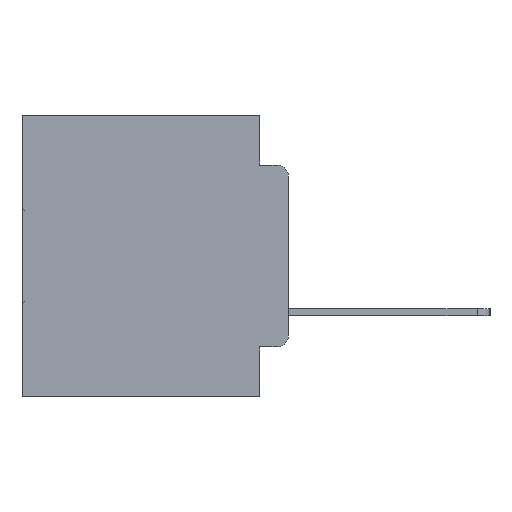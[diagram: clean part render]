
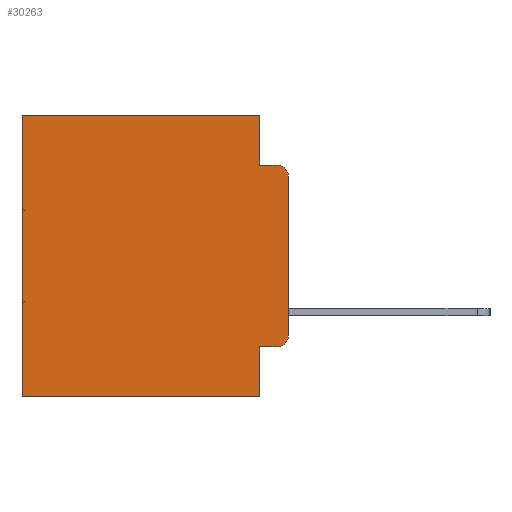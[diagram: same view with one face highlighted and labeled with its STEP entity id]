
A CAD part, left-side view. The second image highlights one B-rep face of the part: STEP entity #30263.
In plain terms, the highlighted planar face has unit normal (-1, 0, 0).
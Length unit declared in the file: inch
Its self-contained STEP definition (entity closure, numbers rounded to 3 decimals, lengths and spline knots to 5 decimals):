
#615 = ORIENTED_EDGE ( 'NONE', *, *, #15617, .T. ) ;
#958 = CARTESIAN_POINT ( 'NONE',  ( 0.298, 0.051, -0.5 ) ) ;
#1130 = VERTEX_POINT ( 'NONE', #10493 ) ;
#1431 = DIRECTION ( 'NONE',  ( 0., -1., 0. ) ) ;
#2017 = EDGE_CURVE ( 'NONE', #1130, #23498, #22075, .T. ) ;
#2206 = ORIENTED_EDGE ( 'NONE', *, *, #25310, .F. ) ;
#2892 = CARTESIAN_POINT ( 'NONE',  ( 0.298, 0.473, -0.5 ) ) ;
#2958 = LINE ( 'NONE', #23111, #21338 ) ;
#3974 = DIRECTION ( 'NONE',  ( 0., 1., 0. ) ) ;
#4320 = VERTEX_POINT ( 'NONE', #21616 ) ;
#4797 = VERTEX_POINT ( 'NONE', #20973 ) ;
#5400 = EDGE_CURVE ( 'NONE', #9654, #25665, #5758, .T. ) ;
#5598 = LINE ( 'NONE', #24920, #23890 ) ;
#5651 = ORIENTED_EDGE ( 'NONE', *, *, #16814, .T. ) ;
#5758 = LINE ( 'NONE', #22285, #17746 ) ;
#5810 = LINE ( 'NONE', #27133, #11495 ) ;
#5849 = DIRECTION ( 'NONE',  ( 0., 0., -1. ) ) ;
#6134 = LINE ( 'NONE', #29048, #24399 ) ;
#6299 = EDGE_CURVE ( 'NONE', #27684, #7325, #24722, .T. ) ;
#7325 = VERTEX_POINT ( 'NONE', #17608 ) ;
#7458 = EDGE_CURVE ( 'NONE', #14294, #4320, #10223, .T. ) ;
#7907 = ORIENTED_EDGE ( 'NONE', *, *, #7458, .F. ) ;
#7931 = EDGE_CURVE ( 'NONE', #11398, #27684, #5598, .T. ) ;
#8004 = DIRECTION ( 'NONE',  ( 0., 0., -1. ) ) ;
#8019 = CARTESIAN_POINT ( 'NONE',  ( 0.298, 0., -0.1085 ) ) ;
#8053 = EDGE_CURVE ( 'NONE', #4797, #4320, #20947, .T. ) ;
#8425 = DIRECTION ( 'NONE',  ( 0., 0., -1. ) ) ;
#9654 = VERTEX_POINT ( 'NONE', #12710 ) ;
#10223 = LINE ( 'NONE', #20423, #28418 ) ;
#10296 = EDGE_LOOP ( 'NONE', ( #7907, #615, #12493, #17296, #15074, #13600, #2206, #22820, #5651, #21004 ) ) ;
#10493 = CARTESIAN_POINT ( 'NONE',  ( 0.298, 0.051, -0.4115 ) ) ;
#10593 = DIRECTION ( 'NONE',  ( -1., 0., 0. ) ) ;
#10696 = AXIS2_PLACEMENT_3D ( 'NONE', #27772, #13616, #30148 ) ;
#11390 = VECTOR ( 'NONE', #1431, 39.37008 ) ;
#11398 = VERTEX_POINT ( 'NONE', #12639 ) ;
#11495 = VECTOR ( 'NONE', #22474, 39.37008 ) ;
#11769 = PLANE ( 'NONE',  #27944 ) ;
#11866 = DIRECTION ( 'NONE',  ( 0., 0., -1. ) ) ;
#12493 = ORIENTED_EDGE ( 'NONE', *, *, #6299, .F. ) ;
#12639 = CARTESIAN_POINT ( 'NONE',  ( 0.298, 0.051, 0. ) ) ;
#12710 = CARTESIAN_POINT ( 'NONE',  ( 0.298, 0.473, 0. ) ) ;
#13374 = CARTESIAN_POINT ( 'NONE',  ( 0.298, 0.051, -0.0885 ) ) ;
#13600 = ORIENTED_EDGE ( 'NONE', *, *, #5400, .T. ) ;
#13616 = DIRECTION ( 'NONE',  ( -1., 0., 0. ) ) ;
#13656 = FACE_OUTER_BOUND ( 'NONE', #10296, .T. ) ;
#14294 = VERTEX_POINT ( 'NONE', #8019 ) ;
#15020 = VECTOR ( 'NONE', #8425, 39.37008 ) ;
#15035 = AXIS2_PLACEMENT_3D ( 'NONE', #24785, #10593, #27182 ) ;
#15074 = ORIENTED_EDGE ( 'NONE', *, *, #19299, .T. ) ;
#15617 = EDGE_CURVE ( 'NONE', #14294, #7325, #23015, .T. ) ;
#16814 = EDGE_CURVE ( 'NONE', #1130, #4797, #6134, .T. ) ;
#17296 = ORIENTED_EDGE ( 'NONE', *, *, #7931, .F. ) ;
#17608 = CARTESIAN_POINT ( 'NONE',  ( 0.298, 0.02, -0.0885 ) ) ;
#17746 = VECTOR ( 'NONE', #8004, 39.37008 ) ;
#18894 = CARTESIAN_POINT ( 'NONE',  ( 0.298, 0., 0. ) ) ;
#19299 = EDGE_CURVE ( 'NONE', #11398, #9654, #5810, .T. ) ;
#20423 = CARTESIAN_POINT ( 'NONE',  ( 0.298, 0., 0. ) ) ;
#20947 = CIRCLE ( 'NONE', #10696, 0.02 ) ;
#20973 = CARTESIAN_POINT ( 'NONE',  ( 0.298, 0.02, -0.4115 ) ) ;
#21004 = ORIENTED_EDGE ( 'NONE', *, *, #8053, .T. ) ;
#21338 = VECTOR ( 'NONE', #3974, 39.37008 ) ;
#21616 = CARTESIAN_POINT ( 'NONE',  ( 0.298, 0., -0.3915 ) ) ;
#22075 = LINE ( 'NONE', #25360, #15020 ) ;
#22285 = CARTESIAN_POINT ( 'NONE',  ( 0.298, 0.473, 0. ) ) ;
#22474 = DIRECTION ( 'NONE',  ( 0., 1., 0. ) ) ;
#22686 = DIRECTION ( 'NONE',  ( 0., 0., -1. ) ) ;
#22820 = ORIENTED_EDGE ( 'NONE', *, *, #2017, .F. ) ;
#23015 = CIRCLE ( 'NONE', #15035, 0.02 ) ;
#23053 = CARTESIAN_POINT ( 'NONE',  ( 0.298, 0.051, -0.0885 ) ) ;
#23111 = CARTESIAN_POINT ( 'NONE',  ( 0.298, 0., -0.5 ) ) ;
#23498 = VERTEX_POINT ( 'NONE', #958 ) ;
#23890 = VECTOR ( 'NONE', #5849, 39.37008 ) ;
#24399 = VECTOR ( 'NONE', #26647, 39.37008 ) ;
#24722 = LINE ( 'NONE', #23053, #11390 ) ;
#24785 = CARTESIAN_POINT ( 'NONE',  ( 0.298, 0.02, -0.1085 ) ) ;
#24920 = CARTESIAN_POINT ( 'NONE',  ( 0.298, 0.051, 0. ) ) ;
#25310 = EDGE_CURVE ( 'NONE', #23498, #25665, #2958, .T. ) ;
#25360 = CARTESIAN_POINT ( 'NONE',  ( 0.298, 0.051, 0. ) ) ;
#25665 = VERTEX_POINT ( 'NONE', #2892 ) ;
#26054 = DIRECTION ( 'NONE',  ( 1., 0., 0. ) ) ;
#26647 = DIRECTION ( 'NONE',  ( 0., -1., 0. ) ) ;
#27133 = CARTESIAN_POINT ( 'NONE',  ( 0.298, 0., 0. ) ) ;
#27182 = DIRECTION ( 'NONE',  ( 0., 0., -1. ) ) ;
#27684 = VERTEX_POINT ( 'NONE', #13374 ) ;
#27772 = CARTESIAN_POINT ( 'NONE',  ( 0.298, 0.02, -0.3915 ) ) ;
#27944 = AXIS2_PLACEMENT_3D ( 'NONE', #18894, #26054, #11866 ) ;
#28418 = VECTOR ( 'NONE', #22686, 39.37008 ) ;
#29048 = CARTESIAN_POINT ( 'NONE',  ( 0.298, 0.051, -0.4115 ) ) ;
#30148 = DIRECTION ( 'NONE',  ( 0., 0., -1. ) ) ;
#30263 = ADVANCED_FACE ( 'NONE', ( #13656 ), #11769, .F. ) ;
